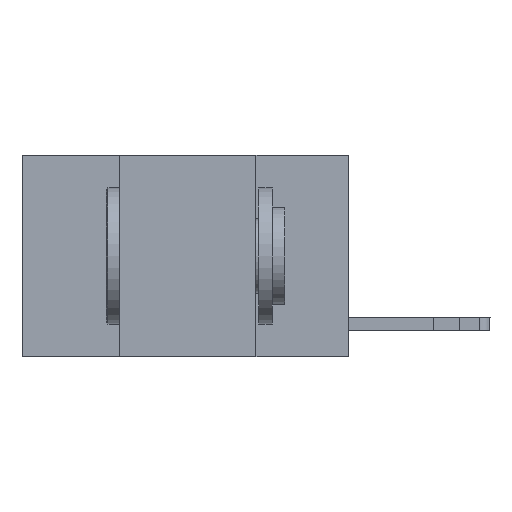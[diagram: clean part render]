
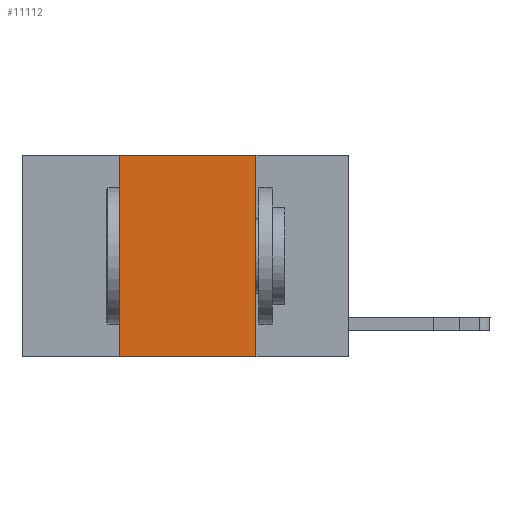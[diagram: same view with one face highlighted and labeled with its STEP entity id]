
A CAD part, left-side view. The second image highlights one B-rep face of the part: STEP entity #11112.
In plain terms, the highlighted planar face has unit normal (-1, 0, 0).
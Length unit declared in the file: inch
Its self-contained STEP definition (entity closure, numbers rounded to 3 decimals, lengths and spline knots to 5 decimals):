
#210 = ORIENTED_EDGE ( 'NONE', *, *, #13365, .F. ) ;
#1909 = EDGE_CURVE ( 'NONE', #8622, #13877, #8652, .T. ) ;
#3027 = CARTESIAN_POINT ( 'NONE',  ( 0., 0.17, -0.37 ) ) ;
#3697 = FACE_OUTER_BOUND ( 'NONE', #11209, .T. ) ;
#3816 = VERTEX_POINT ( 'NONE', #3027 ) ;
#4640 = DIRECTION ( 'NONE',  ( 0., 0., 1. ) ) ;
#4909 = VECTOR ( 'NONE', #7245, 39.37008 ) ;
#5428 = CARTESIAN_POINT ( 'NONE',  ( 0., 0.6, 0. ) ) ;
#5870 = ORIENTED_EDGE ( 'NONE', *, *, #1909, .F. ) ;
#6534 = AXIS2_PLACEMENT_3D ( 'NONE', #5428, #6862, #16591 ) ;
#6814 = CARTESIAN_POINT ( 'NONE',  ( 0., 0.6, 0. ) ) ;
#6862 = DIRECTION ( 'NONE',  ( 1., 0., 0. ) ) ;
#7245 = DIRECTION ( 'NONE',  ( 0., -1., 0. ) ) ;
#8035 = VECTOR ( 'NONE', #17750, 39.37008 ) ;
#8622 = VERTEX_POINT ( 'NONE', #17257 ) ;
#8633 = VERTEX_POINT ( 'NONE', #13168 ) ;
#8652 = LINE ( 'NONE', #6814, #4909 ) ;
#9829 = VECTOR ( 'NONE', #4640, 39.37008 ) ;
#11112 = ADVANCED_FACE ( 'NONE', ( #3697 ), #13808, .F. ) ;
#11209 = EDGE_LOOP ( 'NONE', ( #14324, #5870, #210, #17168 ) ) ;
#11623 = CARTESIAN_POINT ( 'NONE',  ( 0., 0.42, 0. ) ) ;
#11757 = LINE ( 'NONE', #15019, #8035 ) ;
#12972 = VECTOR ( 'NONE', #14267, 39.37008 ) ;
#13168 = CARTESIAN_POINT ( 'NONE',  ( 0., 0.42, -0.37 ) ) ;
#13365 = EDGE_CURVE ( 'NONE', #8633, #8622, #13529, .T. ) ;
#13529 = LINE ( 'NONE', #11623, #9829 ) ;
#13808 = PLANE ( 'NONE',  #6534 ) ;
#13877 = VERTEX_POINT ( 'NONE', #16981 ) ;
#14267 = DIRECTION ( 'NONE',  ( 0., -1., 0. ) ) ;
#14294 = EDGE_CURVE ( 'NONE', #13877, #3816, #11757, .T. ) ;
#14324 = ORIENTED_EDGE ( 'NONE', *, *, #14294, .F. ) ;
#15019 = CARTESIAN_POINT ( 'NONE',  ( 0., 0.17, 0. ) ) ;
#16591 = DIRECTION ( 'NONE',  ( 0., 0., -1. ) ) ;
#16641 = LINE ( 'NONE', #17035, #12972 ) ;
#16981 = CARTESIAN_POINT ( 'NONE',  ( 0., 0.17, 0. ) ) ;
#17035 = CARTESIAN_POINT ( 'NONE',  ( 0., 0.6, -0.37 ) ) ;
#17168 = ORIENTED_EDGE ( 'NONE', *, *, #17404, .T. ) ;
#17257 = CARTESIAN_POINT ( 'NONE',  ( 0., 0.42, 0. ) ) ;
#17404 = EDGE_CURVE ( 'NONE', #8633, #3816, #16641, .T. ) ;
#17750 = DIRECTION ( 'NONE',  ( 0., 0., -1. ) ) ;
